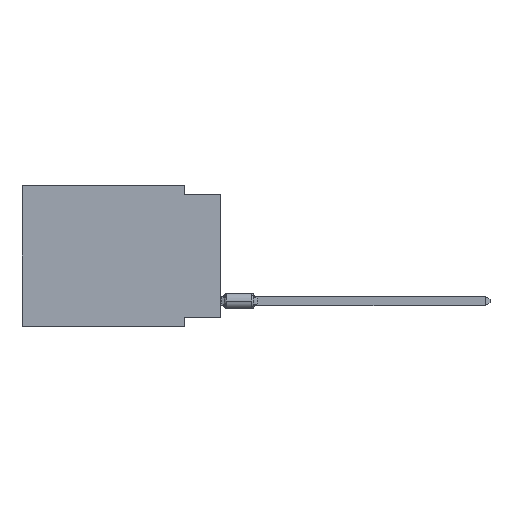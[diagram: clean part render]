
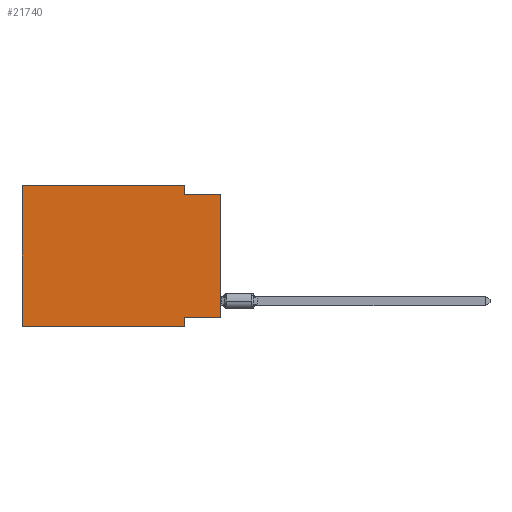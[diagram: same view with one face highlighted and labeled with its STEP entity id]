
A CAD part, left-side view. The second image highlights one B-rep face of the part: STEP entity #21740.
In plain terms, the highlighted planar face has unit normal (-1, 0, 0).
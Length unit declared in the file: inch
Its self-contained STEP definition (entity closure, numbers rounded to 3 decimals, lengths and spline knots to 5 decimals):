
#343 = EDGE_CURVE ( 'NONE', #39300, #37850, #17004, .T. ) ;
#2499 = CARTESIAN_POINT ( 'NONE',  ( 0., 0.55, -0.39 ) ) ;
#3727 = DIRECTION ( 'NONE',  ( 0., -1., 0. ) ) ;
#3739 = VECTOR ( 'NONE', #3727, 39.37008 ) ;
#4732 = VECTOR ( 'NONE', #17781, 39.37008 ) ;
#4992 = CARTESIAN_POINT ( 'NONE',  ( 0., 0.55, 0. ) ) ;
#5428 = ORIENTED_EDGE ( 'NONE', *, *, #343, .F. ) ;
#6560 = CARTESIAN_POINT ( 'NONE',  ( 0., 0.55, 0. ) ) ;
#6711 = EDGE_CURVE ( 'NONE', #26451, #19621, #22316, .T. ) ;
#6791 = LINE ( 'NONE', #7423, #8766 ) ;
#7207 = DIRECTION ( 'NONE',  ( 0., 1., 0. ) ) ;
#7423 = CARTESIAN_POINT ( 'NONE',  ( 0., 0., -0.365 ) ) ;
#7442 = PLANE ( 'NONE',  #20628 ) ;
#7443 = DIRECTION ( 'NONE',  ( 0., 0., -1. ) ) ;
#7570 = CARTESIAN_POINT ( 'NONE',  ( 0., 0.1, -0.39 ) ) ;
#8187 = VERTEX_POINT ( 'NONE', #12296 ) ;
#8766 = VECTOR ( 'NONE', #7207, 39.37008 ) ;
#10649 = LINE ( 'NONE', #6560, #3739 ) ;
#10952 = ORIENTED_EDGE ( 'NONE', *, *, #6711, .T. ) ;
#11123 = CARTESIAN_POINT ( 'NONE',  ( 0., 0., -0.365 ) ) ;
#12296 = CARTESIAN_POINT ( 'NONE',  ( 0., 0., -0.025 ) ) ;
#12833 = ORIENTED_EDGE ( 'NONE', *, *, #22891, .F. ) ;
#14442 = DIRECTION ( 'NONE',  ( 0., 0., 1. ) ) ;
#14861 = ORIENTED_EDGE ( 'NONE', *, *, #38759, .F. ) ;
#14936 = CARTESIAN_POINT ( 'NONE',  ( 0., 0.55, 0. ) ) ;
#15182 = ORIENTED_EDGE ( 'NONE', *, *, #16346, .F. ) ;
#16295 = CARTESIAN_POINT ( 'NONE',  ( 0., 0.1, -0.025 ) ) ;
#16346 = EDGE_CURVE ( 'NONE', #22944, #39300, #10649, .T. ) ;
#17004 = LINE ( 'NONE', #27210, #18089 ) ;
#17124 = VECTOR ( 'NONE', #28731, 39.37008 ) ;
#17781 = DIRECTION ( 'NONE',  ( 0., 0., -1. ) ) ;
#18089 = VECTOR ( 'NONE', #7443, 39.37008 ) ;
#18231 = DIRECTION ( 'NONE',  ( 1., 0., 0. ) ) ;
#18241 = CARTESIAN_POINT ( 'NONE',  ( 0., 0.1, -0.365 ) ) ;
#18749 = EDGE_CURVE ( 'NONE', #26658, #29592, #6791, .T. ) ;
#19170 = CARTESIAN_POINT ( 'NONE',  ( 0., 0., 0. ) ) ;
#19203 = LINE ( 'NONE', #25939, #29157 ) ;
#19621 = VERTEX_POINT ( 'NONE', #34998 ) ;
#20628 = AXIS2_PLACEMENT_3D ( 'NONE', #4992, #18231, #38235 ) ;
#21740 = ADVANCED_FACE ( 'NONE', ( #30669 ), #7442, .F. ) ;
#22221 = LINE ( 'NONE', #19170, #17124 ) ;
#22316 = LINE ( 'NONE', #31657, #35931 ) ;
#22891 = EDGE_CURVE ( 'NONE', #29592, #19621, #26529, .T. ) ;
#22944 = VERTEX_POINT ( 'NONE', #14936 ) ;
#25939 = CARTESIAN_POINT ( 'NONE',  ( 0., 0., -0.025 ) ) ;
#26157 = EDGE_CURVE ( 'NONE', #26451, #22944, #40748, .T. ) ;
#26451 = VERTEX_POINT ( 'NONE', #2499 ) ;
#26529 = LINE ( 'NONE', #7570, #4732 ) ;
#26658 = VERTEX_POINT ( 'NONE', #11123 ) ;
#26715 = EDGE_LOOP ( 'NONE', ( #38373, #14861, #5428, #15182, #26728, #10952, #12833, #31796 ) ) ;
#26728 = ORIENTED_EDGE ( 'NONE', *, *, #26157, .F. ) ;
#27210 = CARTESIAN_POINT ( 'NONE',  ( 0., 0.1, 0. ) ) ;
#28731 = DIRECTION ( 'NONE',  ( 0., 0., 1. ) ) ;
#29157 = VECTOR ( 'NONE', #32466, 39.37008 ) ;
#29592 = VERTEX_POINT ( 'NONE', #18241 ) ;
#30669 = FACE_OUTER_BOUND ( 'NONE', #26715, .T. ) ;
#31429 = DIRECTION ( 'NONE',  ( 0., -1., 0. ) ) ;
#31657 = CARTESIAN_POINT ( 'NONE',  ( 0., 0.55, -0.39 ) ) ;
#31796 = ORIENTED_EDGE ( 'NONE', *, *, #18749, .F. ) ;
#32466 = DIRECTION ( 'NONE',  ( 0., -1., 0. ) ) ;
#34961 = EDGE_CURVE ( 'NONE', #26658, #8187, #22221, .T. ) ;
#34998 = CARTESIAN_POINT ( 'NONE',  ( 0., 0.1, -0.39 ) ) ;
#35931 = VECTOR ( 'NONE', #31429, 39.37008 ) ;
#37493 = CARTESIAN_POINT ( 'NONE',  ( 0., 0.55, 0. ) ) ;
#37594 = CARTESIAN_POINT ( 'NONE',  ( 0., 0.1, 0. ) ) ;
#37850 = VERTEX_POINT ( 'NONE', #16295 ) ;
#38235 = DIRECTION ( 'NONE',  ( 0., 0., -1. ) ) ;
#38257 = VECTOR ( 'NONE', #14442, 39.37008 ) ;
#38373 = ORIENTED_EDGE ( 'NONE', *, *, #34961, .T. ) ;
#38759 = EDGE_CURVE ( 'NONE', #37850, #8187, #19203, .T. ) ;
#39300 = VERTEX_POINT ( 'NONE', #37594 ) ;
#40748 = LINE ( 'NONE', #37493, #38257 ) ;
